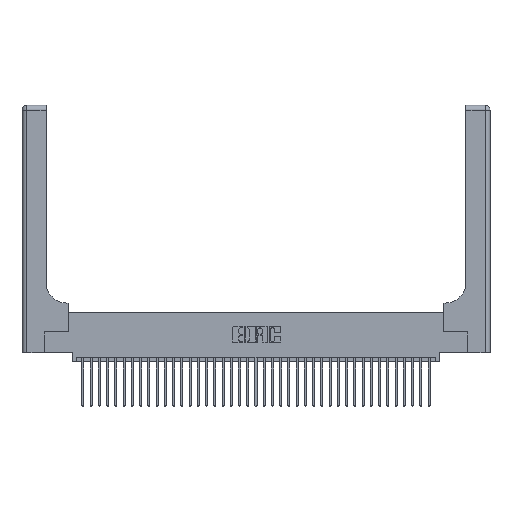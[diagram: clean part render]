
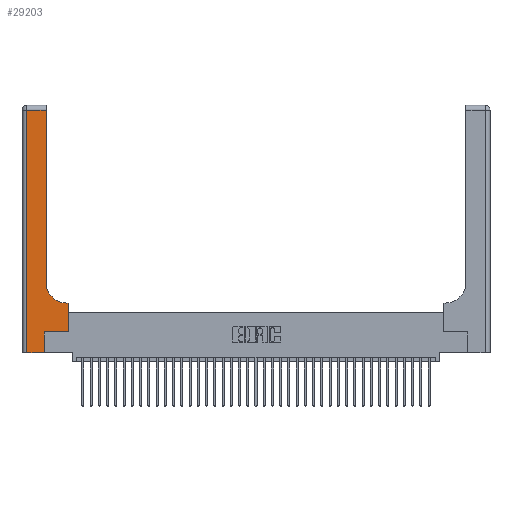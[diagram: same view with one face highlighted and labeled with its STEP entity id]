
A CAD part, top view. The second image highlights one B-rep face of the part: STEP entity #29203.
In plain terms, the highlighted planar face has unit normal (0, 0, 1).
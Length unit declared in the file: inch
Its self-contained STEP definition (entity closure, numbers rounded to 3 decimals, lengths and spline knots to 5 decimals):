
#754 = VECTOR ( 'NONE', #7448, 39.37008 ) ;
#1723 = CARTESIAN_POINT ( 'NONE',  ( 0.269, 0., 0.37 ) ) ;
#1820 = CARTESIAN_POINT ( 'NONE',  ( 0.2915, 0.6, 0.37 ) ) ;
#1867 = PLANE ( 'NONE',  #26031 ) ;
#2083 = CARTESIAN_POINT ( 'NONE',  ( 0.269, 0., 0.37 ) ) ;
#2447 = VECTOR ( 'NONE', #4902, 39.37008 ) ;
#2484 = DIRECTION ( 'NONE',  ( 0., -1., 0. ) ) ;
#2635 = VERTEX_POINT ( 'NONE', #20404 ) ;
#3648 = DIRECTION ( 'NONE',  ( 0., 1., 0. ) ) ;
#3934 = VERTEX_POINT ( 'NONE', #24110 ) ;
#4220 = ORIENTED_EDGE ( 'NONE', *, *, #20615, .T. ) ;
#4568 = EDGE_LOOP ( 'NONE', ( #25714, #4220, #6423, #15544, #18814, #33614, #5967, #5330, #35484 ) ) ;
#4902 = DIRECTION ( 'NONE',  ( 1., 0., 0. ) ) ;
#5244 = VERTEX_POINT ( 'NONE', #7468 ) ;
#5330 = ORIENTED_EDGE ( 'NONE', *, *, #24235, .T. ) ;
#5967 = ORIENTED_EDGE ( 'NONE', *, *, #19348, .T. ) ;
#6093 = VERTEX_POINT ( 'NONE', #10970 ) ;
#6423 = ORIENTED_EDGE ( 'NONE', *, *, #7470, .T. ) ;
#6522 = EDGE_CURVE ( 'NONE', #36327, #6093, #23737, .T. ) ;
#6537 = CARTESIAN_POINT ( 'NONE',  ( 0.2915, 3., 0.37 ) ) ;
#6792 = VECTOR ( 'NONE', #26510, 39.37008 ) ;
#7448 = DIRECTION ( 'NONE',  ( 0., 1., 0. ) ) ;
#7468 = CARTESIAN_POINT ( 'NONE',  ( 0.269, 0.25, 0.37 ) ) ;
#7470 = EDGE_CURVE ( 'NONE', #3934, #21941, #17558, .T. ) ;
#7613 = AXIS2_PLACEMENT_3D ( 'NONE', #25697, #28599, #8084 ) ;
#8084 = DIRECTION ( 'NONE',  ( 1., 0., 0. ) ) ;
#9752 = VERTEX_POINT ( 'NONE', #27225 ) ;
#9885 = VERTEX_POINT ( 'NONE', #20129 ) ;
#10432 = FACE_OUTER_BOUND ( 'NONE', #4568, .T. ) ;
#10617 = VECTOR ( 'NONE', #19504, 39.37008 ) ;
#10897 = CARTESIAN_POINT ( 'NONE',  ( 0.06, 0., 0.37 ) ) ;
#10970 = CARTESIAN_POINT ( 'NONE',  ( 0.2915, 2.94, 0.37 ) ) ;
#11454 = DIRECTION ( 'NONE',  ( 0., 1., 0. ) ) ;
#11519 = VECTOR ( 'NONE', #3648, 39.37008 ) ;
#12585 = CARTESIAN_POINT ( 'NONE',  ( 0., 0., 0.37 ) ) ;
#12794 = EDGE_CURVE ( 'NONE', #9752, #36327, #30545, .T. ) ;
#14475 = DIRECTION ( 'NONE',  ( -1., 0., 0. ) ) ;
#14784 = LINE ( 'NONE', #1820, #6792 ) ;
#14855 = LINE ( 'NONE', #12585, #10617 ) ;
#15544 = ORIENTED_EDGE ( 'NONE', *, *, #32831, .T. ) ;
#15568 = LINE ( 'NONE', #2083, #38592 ) ;
#16623 = VECTOR ( 'NONE', #2484, 39.37008 ) ;
#17558 = LINE ( 'NONE', #23398, #16623 ) ;
#18814 = ORIENTED_EDGE ( 'NONE', *, *, #25660, .T. ) ;
#19149 = CARTESIAN_POINT ( 'NONE',  ( 0.5585, 0.25, 0.37 ) ) ;
#19348 = EDGE_CURVE ( 'NONE', #9885, #2635, #31387, .T. ) ;
#19504 = DIRECTION ( 'NONE',  ( 1., 0., 0. ) ) ;
#20129 = CARTESIAN_POINT ( 'NONE',  ( 0.5585, 0.25, 0.37 ) ) ;
#20404 = CARTESIAN_POINT ( 'NONE',  ( 0.5585, 0.6, 0.37 ) ) ;
#20615 = EDGE_CURVE ( 'NONE', #6093, #3934, #28445, .T. ) ;
#21941 = VERTEX_POINT ( 'NONE', #10897 ) ;
#23153 = VERTEX_POINT ( 'NONE', #1723 ) ;
#23294 = VECTOR ( 'NONE', #31165, 39.37008 ) ;
#23398 = CARTESIAN_POINT ( 'NONE',  ( 0.06, 3., 0.37 ) ) ;
#23737 = LINE ( 'NONE', #6537, #11519 ) ;
#24110 = CARTESIAN_POINT ( 'NONE',  ( 0.06, 2.94, 0.37 ) ) ;
#24235 = EDGE_CURVE ( 'NONE', #2635, #9752, #14784, .T. ) ;
#25660 = EDGE_CURVE ( 'NONE', #23153, #5244, #15568, .T. ) ;
#25697 = CARTESIAN_POINT ( 'NONE',  ( 0.5415, 0.85, 0.37 ) ) ;
#25714 = ORIENTED_EDGE ( 'NONE', *, *, #6522, .T. ) ;
#26031 = AXIS2_PLACEMENT_3D ( 'NONE', #38932, #29860, #14475 ) ;
#26510 = DIRECTION ( 'NONE',  ( -1., 0., 0. ) ) ;
#27225 = CARTESIAN_POINT ( 'NONE',  ( 0.5415, 0.6, 0.37 ) ) ;
#27393 = LINE ( 'NONE', #28426, #2447 ) ;
#28144 = CARTESIAN_POINT ( 'NONE',  ( 0., 2.94, 0.37 ) ) ;
#28426 = CARTESIAN_POINT ( 'NONE',  ( 0.269, 0.25, 0.37 ) ) ;
#28445 = LINE ( 'NONE', #28144, #23294 ) ;
#28599 = DIRECTION ( 'NONE',  ( 0., 0., -1. ) ) ;
#29047 = EDGE_CURVE ( 'NONE', #5244, #9885, #27393, .T. ) ;
#29203 = ADVANCED_FACE ( 'NONE', ( #10432 ), #1867, .F. ) ;
#29860 = DIRECTION ( 'NONE',  ( 0., 0., -1. ) ) ;
#30545 = CIRCLE ( 'NONE', #7613, 0.25 ) ;
#31165 = DIRECTION ( 'NONE',  ( -1., 0., 0. ) ) ;
#31387 = LINE ( 'NONE', #19149, #754 ) ;
#32831 = EDGE_CURVE ( 'NONE', #21941, #23153, #14855, .T. ) ;
#32885 = CARTESIAN_POINT ( 'NONE',  ( 0.2915, 0.85, 0.37 ) ) ;
#33614 = ORIENTED_EDGE ( 'NONE', *, *, #29047, .T. ) ;
#35484 = ORIENTED_EDGE ( 'NONE', *, *, #12794, .T. ) ;
#36327 = VERTEX_POINT ( 'NONE', #32885 ) ;
#38592 = VECTOR ( 'NONE', #11454, 39.37008 ) ;
#38932 = CARTESIAN_POINT ( 'NONE',  ( 0., 3., 0.37 ) ) ;
